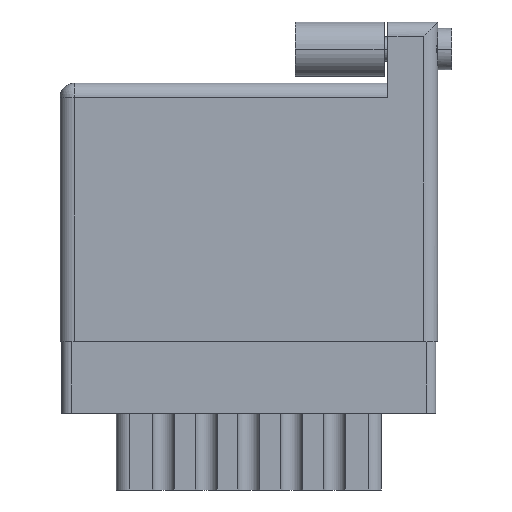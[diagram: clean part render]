
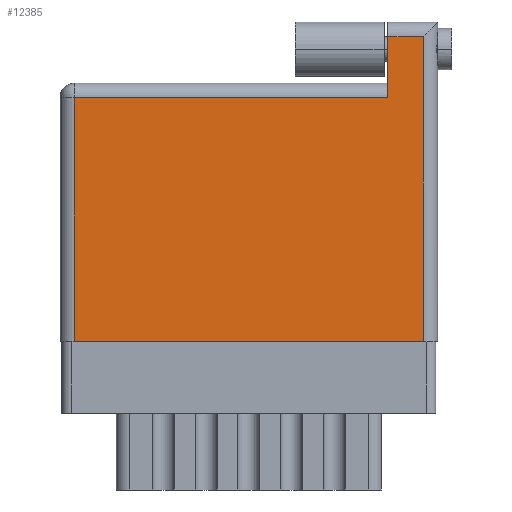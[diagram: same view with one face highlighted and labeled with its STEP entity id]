
A CAD part, front view. The second image highlights one B-rep face of the part: STEP entity #12385.
In plain terms, the highlighted face is planar.
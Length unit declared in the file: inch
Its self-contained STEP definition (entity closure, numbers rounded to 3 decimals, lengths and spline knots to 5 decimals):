
#263 = VECTOR ( 'NONE', #14960, 39.37008 ) ;
#537 = CARTESIAN_POINT ( 'NONE',  ( 1.15, 1.12, 0. ) ) ;
#756 = VERTEX_POINT ( 'NONE', #14502 ) ;
#1200 = VECTOR ( 'NONE', #20862, 39.37008 ) ;
#1780 = EDGE_LOOP ( 'NONE', ( #23282, #2330, #15191, #6198, #20460, #20815 ) ) ;
#1951 = VERTEX_POINT ( 'NONE', #10702 ) ;
#2330 = ORIENTED_EDGE ( 'NONE', *, *, #11654, .T. ) ;
#2381 = LINE ( 'NONE', #537, #11622 ) ;
#4011 = VERTEX_POINT ( 'NONE', #14372 ) ;
#4099 = LINE ( 'NONE', #17794, #20964 ) ;
#4203 = CARTESIAN_POINT ( 'NONE',  ( 1.15, 0.856, 0. ) ) ;
#5922 = DIRECTION ( 'NONE',  ( 0., 1., 0. ) ) ;
#6017 = DIRECTION ( 'NONE',  ( 0., -1., 0. ) ) ;
#6198 = ORIENTED_EDGE ( 'NONE', *, *, #23562, .T. ) ;
#7405 = DIRECTION ( 'NONE',  ( -1., 0., 0. ) ) ;
#9868 = EDGE_CURVE ( 'NONE', #756, #25498, #4099, .T. ) ;
#10685 = CARTESIAN_POINT ( 'NONE',  ( 0.05, 0., 0. ) ) ;
#10702 = CARTESIAN_POINT ( 'NONE',  ( 1.275, 0., 0. ) ) ;
#10994 = CARTESIAN_POINT ( 'NONE',  ( 0., 1.07, 0. ) ) ;
#11566 = CARTESIAN_POINT ( 'NONE',  ( 0., 0.906, 0. ) ) ;
#11622 = VECTOR ( 'NONE', #6017, 39.37008 ) ;
#11654 = EDGE_CURVE ( 'NONE', #1951, #13546, #17801, .T. ) ;
#12385 = ADVANCED_FACE ( 'NONE', ( #23329 ), #17326, .F. ) ;
#12726 = CARTESIAN_POINT ( 'NONE',  ( 0., 0.856, 0. ) ) ;
#13219 = DIRECTION ( 'NONE',  ( -1., 0., 0. ) ) ;
#13408 = DIRECTION ( 'NONE',  ( 0., 0., -1. ) ) ;
#13546 = VERTEX_POINT ( 'NONE', #22662 ) ;
#14372 = CARTESIAN_POINT ( 'NONE',  ( 1.15, 1.07, 0. ) ) ;
#14452 = LINE ( 'NONE', #12726, #263 ) ;
#14502 = CARTESIAN_POINT ( 'NONE',  ( 0.05, 0.856, 0. ) ) ;
#14948 = AXIS2_PLACEMENT_3D ( 'NONE', #11566, #13408, #7405 ) ;
#14960 = DIRECTION ( 'NONE',  ( -1., 0., 0. ) ) ;
#15191 = ORIENTED_EDGE ( 'NONE', *, *, #19439, .T. ) ;
#16832 = LINE ( 'NONE', #24799, #1200 ) ;
#17326 = PLANE ( 'NONE',  #14948 ) ;
#17794 = CARTESIAN_POINT ( 'NONE',  ( 0.05, 0., 0. ) ) ;
#17801 = LINE ( 'NONE', #23803, #21898 ) ;
#18713 = VERTEX_POINT ( 'NONE', #4203 ) ;
#19439 = EDGE_CURVE ( 'NONE', #13546, #4011, #20789, .T. ) ;
#19449 = VECTOR ( 'NONE', #13219, 39.37008 ) ;
#20225 = EDGE_CURVE ( 'NONE', #18713, #756, #14452, .T. ) ;
#20460 = ORIENTED_EDGE ( 'NONE', *, *, #20225, .T. ) ;
#20789 = LINE ( 'NONE', #10994, #19449 ) ;
#20815 = ORIENTED_EDGE ( 'NONE', *, *, #9868, .T. ) ;
#20862 = DIRECTION ( 'NONE',  ( 1., 0., 0. ) ) ;
#20964 = VECTOR ( 'NONE', #23921, 39.37008 ) ;
#21898 = VECTOR ( 'NONE', #5922, 39.37008 ) ;
#22662 = CARTESIAN_POINT ( 'NONE',  ( 1.275, 1.07, 0. ) ) ;
#23038 = EDGE_CURVE ( 'NONE', #25498, #1951, #16832, .T. ) ;
#23282 = ORIENTED_EDGE ( 'NONE', *, *, #23038, .T. ) ;
#23329 = FACE_OUTER_BOUND ( 'NONE', #1780, .T. ) ;
#23562 = EDGE_CURVE ( 'NONE', #4011, #18713, #2381, .T. ) ;
#23803 = CARTESIAN_POINT ( 'NONE',  ( 1.275, 1.12, 0. ) ) ;
#23921 = DIRECTION ( 'NONE',  ( 0., -1., 0. ) ) ;
#24799 = CARTESIAN_POINT ( 'NONE',  ( 0., 0., 0. ) ) ;
#25498 = VERTEX_POINT ( 'NONE', #10685 ) ;
